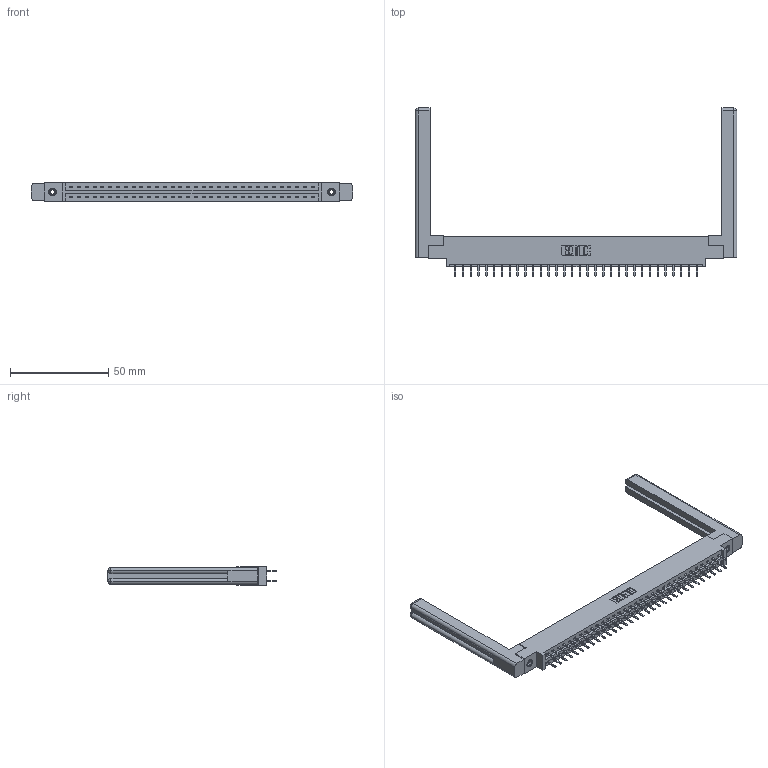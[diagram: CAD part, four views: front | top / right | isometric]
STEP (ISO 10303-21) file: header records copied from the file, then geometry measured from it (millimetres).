
FILE_DESCRIPTION (( 'STEP AP203' ), '1' );
FILE_NAME ('337-064-520-858.STEP', '2019-10-11T23:27:44', ( '' ), ( '' ), 'SwSTEP 2.0', 'SolidWorks 2016', '' );
FILE_SCHEMA (( 'CONFIG_CONTROL_DESIGN' ));
Length unit declared in the file: inch
Products named in the file (5): 307-220-058; 345-250-001_345-250-001-102; 345-292-001_345-293-120; 337 Part_0.170 Offset - 0.156 Dia-TI; 337-064-520-858
Assembly tree (69 placements, depth 2):
  337-064-520-858
    337 Part_0.170 Offset - 0.156 Dia-TI
    345-292-001_345-293-120  x64
    345-250-001_345-250-001-102  x2
    307-220-058  x2
Bounding box: 163.42 x 85.43 x 9.4 mm (x, y, z)
Volume: 24086.5 mm3; surface area: 24132.6 mm2
Topology: 69 solids, 69 shells, 3972 faces, 11493 edges, 7478 vertices
Faces by surface type: plane 2718, cylinder 1230, cone 12, torus 12
Entity records: 28984 total; most frequent: CARTESIAN_POINT 4913, ORIENTED_EDGE 4776, DIRECTION 4200, EDGE_CURVE 2388, VECTOR 2208, LINE 2208, VERTEX_POINT 1582, AXIS2_PLACEMENT_3D 996
